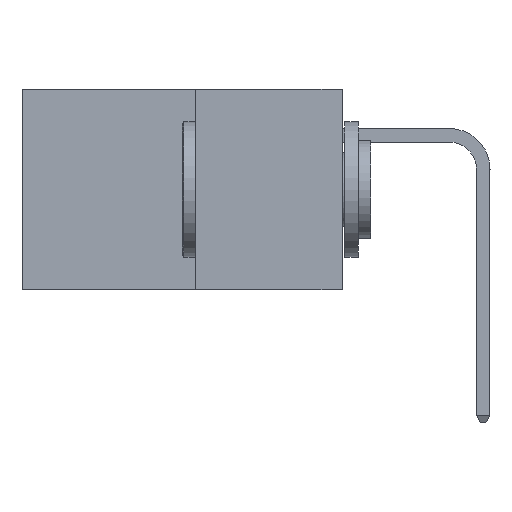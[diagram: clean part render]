
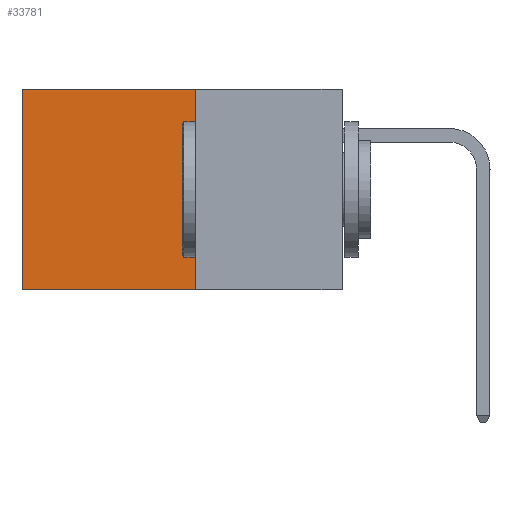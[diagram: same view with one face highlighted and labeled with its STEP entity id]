
A CAD part, left-side view. The second image highlights one B-rep face of the part: STEP entity #33781.
In plain terms, the highlighted planar face has unit normal (-1, 0, 0).
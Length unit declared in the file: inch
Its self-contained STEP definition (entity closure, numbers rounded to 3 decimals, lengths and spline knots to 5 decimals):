
#745 = VECTOR ( 'NONE', #23018, 39.37008 ) ;
#1276 = EDGE_CURVE ( 'NONE', #26950, #22066, #14737, .T. ) ;
#2419 = CARTESIAN_POINT ( 'NONE',  ( 0.277, 0.27, 0. ) ) ;
#3584 = CARTESIAN_POINT ( 'NONE',  ( 0.277, 0.27, 0. ) ) ;
#3624 = VERTEX_POINT ( 'NONE', #11358 ) ;
#3740 = CARTESIAN_POINT ( 'NONE',  ( 0.277, 0.59, -0.37 ) ) ;
#3885 = VERTEX_POINT ( 'NONE', #3740 ) ;
#4807 = CARTESIAN_POINT ( 'NONE',  ( 0.277, 0.27, -0.37 ) ) ;
#6695 = LINE ( 'NONE', #3584, #33754 ) ;
#7877 = LINE ( 'NONE', #29865, #28843 ) ;
#8072 = AXIS2_PLACEMENT_3D ( 'NONE', #10372, #28779, #13014 ) ;
#8189 = EDGE_CURVE ( 'NONE', #26950, #3624, #6695, .T. ) ;
#8411 = LINE ( 'NONE', #14717, #19962 ) ;
#8792 = ORIENTED_EDGE ( 'NONE', *, *, #12526, .T. ) ;
#9531 = DIRECTION ( 'NONE',  ( 0., 1., 0. ) ) ;
#10067 = FACE_OUTER_BOUND ( 'NONE', #33951, .T. ) ;
#10372 = CARTESIAN_POINT ( 'NONE',  ( 0.277, 0.27, -0.37 ) ) ;
#10686 = EDGE_CURVE ( 'NONE', #22066, #3885, #8411, .T. ) ;
#11358 = CARTESIAN_POINT ( 'NONE',  ( 0.277, 0.59, 0. ) ) ;
#11512 = DIRECTION ( 'NONE',  ( 0., 1., 0. ) ) ;
#12526 = EDGE_CURVE ( 'NONE', #3624, #3885, #7877, .T. ) ;
#13014 = DIRECTION ( 'NONE',  ( 0., 0., -1. ) ) ;
#13433 = ORIENTED_EDGE ( 'NONE', *, *, #1276, .F. ) ;
#14717 = CARTESIAN_POINT ( 'NONE',  ( 0.277, 0.27, -0.37 ) ) ;
#14737 = LINE ( 'NONE', #4807, #745 ) ;
#16793 = DIRECTION ( 'NONE',  ( 0., 0., -1. ) ) ;
#19962 = VECTOR ( 'NONE', #9531, 39.37008 ) ;
#22066 = VERTEX_POINT ( 'NONE', #24700 ) ;
#22956 = ORIENTED_EDGE ( 'NONE', *, *, #10686, .F. ) ;
#23018 = DIRECTION ( 'NONE',  ( 0., 0., -1. ) ) ;
#24700 = CARTESIAN_POINT ( 'NONE',  ( 0.277, 0.27, -0.37 ) ) ;
#26160 = PLANE ( 'NONE',  #8072 ) ;
#26950 = VERTEX_POINT ( 'NONE', #2419 ) ;
#28779 = DIRECTION ( 'NONE',  ( 1., 0., 0. ) ) ;
#28843 = VECTOR ( 'NONE', #16793, 39.37008 ) ;
#29865 = CARTESIAN_POINT ( 'NONE',  ( 0.277, 0.59, -0.37 ) ) ;
#30247 = ORIENTED_EDGE ( 'NONE', *, *, #8189, .T. ) ;
#33754 = VECTOR ( 'NONE', #11512, 39.37008 ) ;
#33781 = ADVANCED_FACE ( 'NONE', ( #10067 ), #26160, .F. ) ;
#33951 = EDGE_LOOP ( 'NONE', ( #8792, #22956, #13433, #30247 ) ) ;
